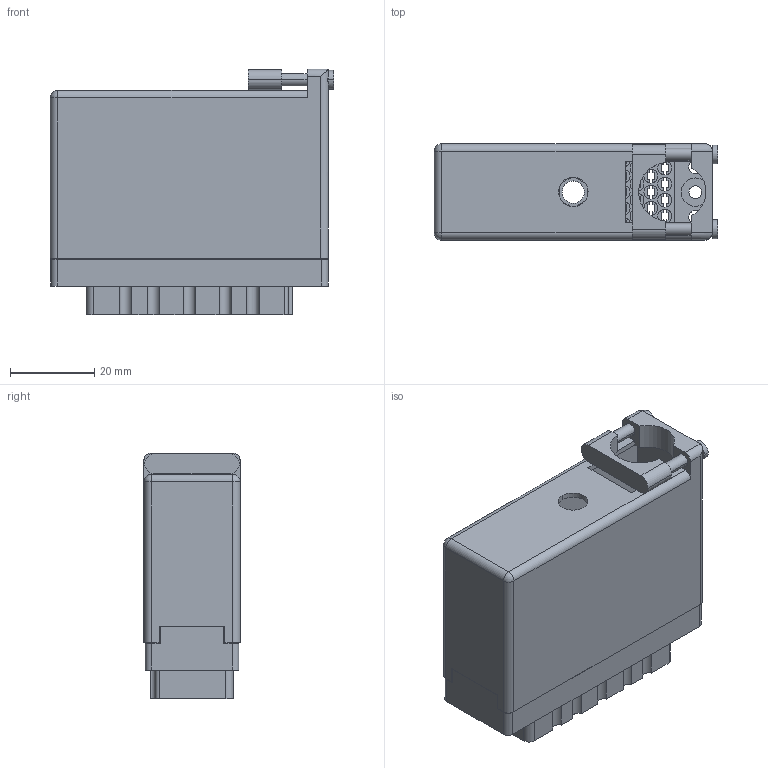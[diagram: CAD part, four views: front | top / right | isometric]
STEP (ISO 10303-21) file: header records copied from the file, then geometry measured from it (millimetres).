
FILE_DESCRIPTION (( 'STEP AP203' ), '1' );
FILE_NAME ('516-056-000-660.STEP', '2020-03-05T20:56:39', ( '' ), ( '' ), 'SwSTEP 2.0', 'SolidWorks 2016', '' );
FILE_SCHEMA (( 'CONFIG_CONTROL_DESIGN' ));
Length unit declared in the file: inch
Products named in the file (3): 516-056-000-660; 516 Part Receptacle_056; 516-230-001_Metal - 056 Top Entry
Assembly tree (2 placements, depth 2):
  516-056-000-660
    516 Part Receptacle_056
    516-230-001_Metal - 056 Top Entry
Bounding box: 67.31 x 22.83 x 58.34 mm (x, y, z)
Volume: 24634.7 mm3; surface area: 36469.5 mm2
Topology: 2 solids, 2 shells, 1329 faces, 3916 edges, 2604 vertices
Faces by surface type: plane 926, cylinder 399, cone 2, sphere 2
Entity records: 44913 total; most frequent: CARTESIAN_POINT 7894, ORIENTED_EDGE 7828, DIRECTION 7598, EDGE_CURVE 3914, VECTOR 2886, LINE 2886, VERTEX_POINT 2604, AXIS2_PLACEMENT_3D 2356
